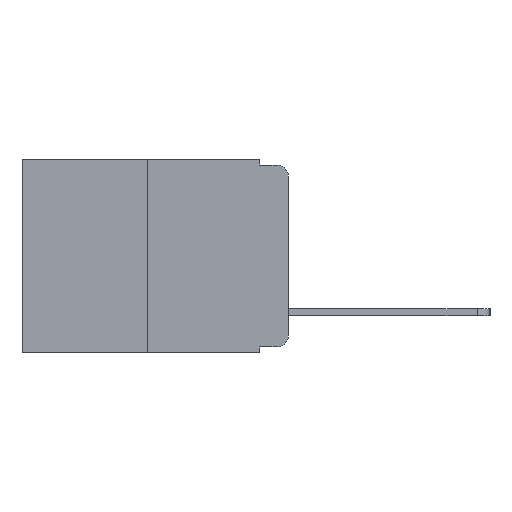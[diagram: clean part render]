
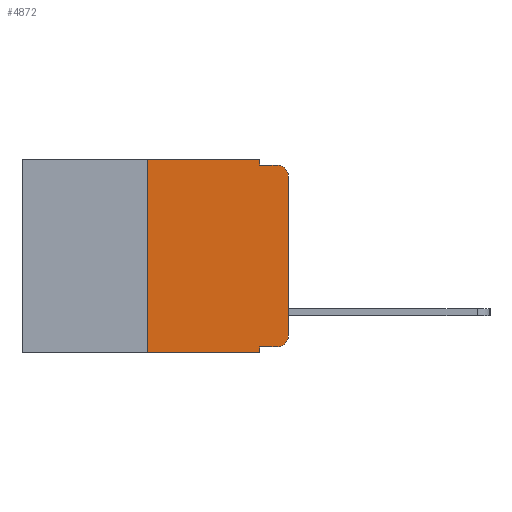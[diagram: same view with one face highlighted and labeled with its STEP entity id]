
A CAD part, left-side view. The second image highlights one B-rep face of the part: STEP entity #4872.
In plain terms, the highlighted planar face has unit normal (-1, 0, 0).
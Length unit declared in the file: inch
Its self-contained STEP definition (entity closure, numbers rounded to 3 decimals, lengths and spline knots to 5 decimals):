
#348 = ORIENTED_EDGE ( 'NONE', *, *, #7205, .T. ) ;
#349 = VECTOR ( 'NONE', #4128, 39.37008 ) ;
#806 = ORIENTED_EDGE ( 'NONE', *, *, #7293, .F. ) ;
#1263 = DIRECTION ( 'NONE',  ( 0., -1., 0. ) ) ;
#1313 = VECTOR ( 'NONE', #16683, 39.37008 ) ;
#2250 = AXIS2_PLACEMENT_3D ( 'NONE', #11783, #2970, #12053 ) ;
#2653 = ORIENTED_EDGE ( 'NONE', *, *, #7269, .F. ) ;
#2676 = ORIENTED_EDGE ( 'NONE', *, *, #7327, .T. ) ;
#2679 = ORIENTED_EDGE ( 'NONE', *, *, #7241, .T. ) ;
#2808 = ORIENTED_EDGE ( 'NONE', *, *, #7243, .F. ) ;
#2970 = DIRECTION ( 'NONE',  ( -1., 0., 0. ) ) ;
#3294 = VECTOR ( 'NONE', #5117, 39.37008 ) ;
#3295 = ORIENTED_EDGE ( 'NONE', *, *, #10147, .T. ) ;
#3618 = DIRECTION ( 'NONE',  ( 1., 0., 0. ) ) ;
#4010 = VERTEX_POINT ( 'NONE', #16773 ) ;
#4128 = DIRECTION ( 'NONE',  ( 0., -1., 0. ) ) ;
#4872 = ADVANCED_FACE ( 'NONE', ( #6328 ), #14892, .F. ) ;
#5117 = DIRECTION ( 'NONE',  ( 0., 0., -1. ) ) ;
#5910 = DIRECTION ( 'NONE',  ( 0., 0., 1. ) ) ;
#5913 = ORIENTED_EDGE ( 'NONE', *, *, #7900, .F. ) ;
#6026 = CARTESIAN_POINT ( 'NONE',  ( 0., 0.25, -0.343 ) ) ;
#6248 = CARTESIAN_POINT ( 'NONE',  ( 0., 0.051, -0.343 ) ) ;
#6328 = FACE_OUTER_BOUND ( 'NONE', #13079, .T. ) ;
#6425 = VERTEX_POINT ( 'NONE', #11746 ) ;
#6839 = EDGE_CURVE ( 'NONE', #9917, #7075, #12190, .T. ) ;
#7075 = VERTEX_POINT ( 'NONE', #7376 ) ;
#7205 = EDGE_CURVE ( 'NONE', #15464, #9917, #15851, .T. ) ;
#7241 = EDGE_CURVE ( 'NONE', #6425, #15464, #14662, .T. ) ;
#7243 = EDGE_CURVE ( 'NONE', #6425, #17391, #17533, .T. ) ;
#7269 = EDGE_CURVE ( 'NONE', #10694, #15190, #9936, .T. ) ;
#7283 = CARTESIAN_POINT ( 'NONE',  ( 0., 0.25, 0. ) ) ;
#7293 = EDGE_CURVE ( 'NONE', #12912, #4010, #13841, .T. ) ;
#7320 = EDGE_CURVE ( 'NONE', #4010, #10253, #11772, .T. ) ;
#7327 = EDGE_CURVE ( 'NONE', #7075, #10253, #14838, .T. ) ;
#7367 = CARTESIAN_POINT ( 'NONE',  ( 0., 0., -0.313 ) ) ;
#7376 = CARTESIAN_POINT ( 'NONE',  ( 0., 0., -0.03 ) ) ;
#7417 = CARTESIAN_POINT ( 'NONE',  ( 0., 0.051, 0. ) ) ;
#7454 = VECTOR ( 'NONE', #17227, 39.37008 ) ;
#7900 = EDGE_CURVE ( 'NONE', #15190, #12912, #18215, .T. ) ;
#8159 = VECTOR ( 'NONE', #9346, 39.37008 ) ;
#8681 = CARTESIAN_POINT ( 'NONE',  ( 0., 0.02, -0.03 ) ) ;
#9346 = DIRECTION ( 'NONE',  ( 0., 0., 1. ) ) ;
#9732 = CARTESIAN_POINT ( 'NONE',  ( 0., 0.473, 0. ) ) ;
#9917 = VERTEX_POINT ( 'NONE', #7367 ) ;
#9936 = LINE ( 'NONE', #15377, #16387 ) ;
#10121 = DIRECTION ( 'NONE',  ( 0., 0., -1. ) ) ;
#10147 = EDGE_CURVE ( 'NONE', #10694, #17391, #13458, .T. ) ;
#10253 = VERTEX_POINT ( 'NONE', #14800 ) ;
#10694 = VERTEX_POINT ( 'NONE', #6026 ) ;
#10722 = CARTESIAN_POINT ( 'NONE',  ( 0., 0.051, -0.333 ) ) ;
#10899 = ORIENTED_EDGE ( 'NONE', *, *, #6839, .T. ) ;
#11746 = CARTESIAN_POINT ( 'NONE',  ( 0., 0.051, -0.333 ) ) ;
#11772 = LINE ( 'NONE', #17657, #349 ) ;
#11783 = CARTESIAN_POINT ( 'NONE',  ( 0., 0.02, -0.313 ) ) ;
#12053 = DIRECTION ( 'NONE',  ( 0., 0., -1. ) ) ;
#12190 = LINE ( 'NONE', #14416, #8159 ) ;
#12912 = VERTEX_POINT ( 'NONE', #15546 ) ;
#13079 = EDGE_LOOP ( 'NONE', ( #10899, #2676, #14138, #806, #5913, #2653, #3295, #2808, #2679, #348 ) ) ;
#13256 = AXIS2_PLACEMENT_3D ( 'NONE', #9732, #3618, #14346 ) ;
#13288 = CARTESIAN_POINT ( 'NONE',  ( 0., 0.473, -0.343 ) ) ;
#13458 = LINE ( 'NONE', #13288, #16433 ) ;
#13513 = CARTESIAN_POINT ( 'NONE',  ( 0., 0.473, 0. ) ) ;
#13841 = LINE ( 'NONE', #7417, #1313 ) ;
#14138 = ORIENTED_EDGE ( 'NONE', *, *, #7320, .F. ) ;
#14346 = DIRECTION ( 'NONE',  ( 0., 0., -1. ) ) ;
#14416 = CARTESIAN_POINT ( 'NONE',  ( 0., 0., 0. ) ) ;
#14653 = DIRECTION ( 'NONE',  ( 0., -1., 0. ) ) ;
#14662 = LINE ( 'NONE', #10722, #7454 ) ;
#14800 = CARTESIAN_POINT ( 'NONE',  ( 0., 0.02, -0.01 ) ) ;
#14838 = CIRCLE ( 'NONE', #17237, 0.02 ) ;
#14892 = PLANE ( 'NONE',  #13256 ) ;
#15190 = VERTEX_POINT ( 'NONE', #7283 ) ;
#15377 = CARTESIAN_POINT ( 'NONE',  ( 0., 0.25, 0. ) ) ;
#15464 = VERTEX_POINT ( 'NONE', #15899 ) ;
#15546 = CARTESIAN_POINT ( 'NONE',  ( 0., 0.051, 0. ) ) ;
#15851 = CIRCLE ( 'NONE', #2250, 0.02 ) ;
#15899 = CARTESIAN_POINT ( 'NONE',  ( 0., 0.02, -0.333 ) ) ;
#16387 = VECTOR ( 'NONE', #5910, 39.37008 ) ;
#16433 = VECTOR ( 'NONE', #14653, 39.37008 ) ;
#16683 = DIRECTION ( 'NONE',  ( 0., 0., -1. ) ) ;
#16773 = CARTESIAN_POINT ( 'NONE',  ( 0., 0.051, -0.01 ) ) ;
#17085 = VECTOR ( 'NONE', #1263, 39.37008 ) ;
#17227 = DIRECTION ( 'NONE',  ( 0., -1., 0. ) ) ;
#17237 = AXIS2_PLACEMENT_3D ( 'NONE', #8681, #17760, #10121 ) ;
#17340 = CARTESIAN_POINT ( 'NONE',  ( 0., 0.051, 0. ) ) ;
#17391 = VERTEX_POINT ( 'NONE', #6248 ) ;
#17533 = LINE ( 'NONE', #17340, #3294 ) ;
#17657 = CARTESIAN_POINT ( 'NONE',  ( 0., 0.051, -0.01 ) ) ;
#17760 = DIRECTION ( 'NONE',  ( -1., 0., 0. ) ) ;
#18215 = LINE ( 'NONE', #13513, #17085 ) ;
